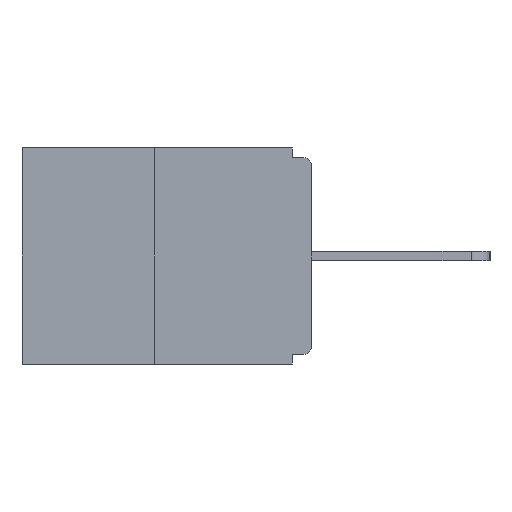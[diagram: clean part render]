
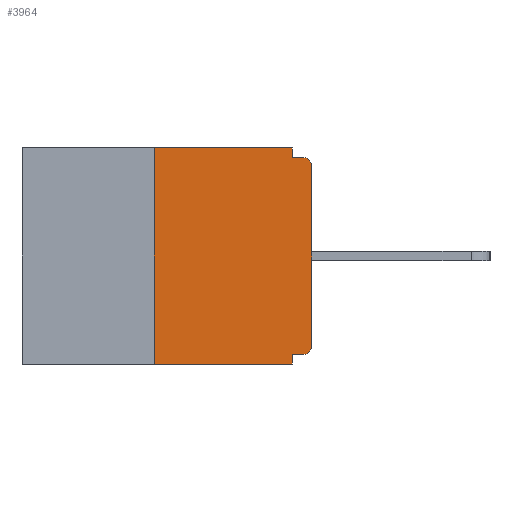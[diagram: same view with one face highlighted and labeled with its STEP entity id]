
A CAD part, left-side view. The second image highlights one B-rep face of the part: STEP entity #3964.
In plain terms, the highlighted planar face has unit normal (-1, 0, 0).
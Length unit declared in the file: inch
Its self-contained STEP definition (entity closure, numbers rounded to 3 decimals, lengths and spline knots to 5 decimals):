
#217 = ORIENTED_EDGE ( 'NONE', *, *, #3717, .T. ) ;
#448 = DIRECTION ( 'NONE',  ( 0., 0., 1. ) ) ;
#612 = VERTEX_POINT ( 'NONE', #13465 ) ;
#772 = LINE ( 'NONE', #8104, #11012 ) ;
#862 = CIRCLE ( 'NONE', #11757, 0.015 ) ;
#958 = CARTESIAN_POINT ( 'NONE',  ( 0., 0., -0.015 ) ) ;
#1286 = VERTEX_POINT ( 'NONE', #6840 ) ;
#1301 = DIRECTION ( 'NONE',  ( 0., -1., 0. ) ) ;
#1333 = CARTESIAN_POINT ( 'NONE',  ( 0., 0.46, 0. ) ) ;
#1517 = ORIENTED_EDGE ( 'NONE', *, *, #14746, .T. ) ;
#1579 = EDGE_CURVE ( 'NONE', #1286, #2035, #12419, .T. ) ;
#2035 = VERTEX_POINT ( 'NONE', #4166 ) ;
#2094 = VECTOR ( 'NONE', #10091, 39.37008 ) ;
#2253 = VERTEX_POINT ( 'NONE', #12683 ) ;
#2357 = LINE ( 'NONE', #7444, #13769 ) ;
#2391 = LINE ( 'NONE', #958, #8960 ) ;
#2914 = ORIENTED_EDGE ( 'NONE', *, *, #11881, .T. ) ;
#3104 = CIRCLE ( 'NONE', #14000, 0.015 ) ;
#3200 = CARTESIAN_POINT ( 'NONE',  ( 0., 0.031, -0.343 ) ) ;
#3345 = DIRECTION ( 'NONE',  ( 0., 0., -1. ) ) ;
#3346 = ORIENTED_EDGE ( 'NONE', *, *, #9229, .F. ) ;
#3465 = DIRECTION ( 'NONE',  ( 0., 0., -1. ) ) ;
#3518 = DIRECTION ( 'NONE',  ( 0., 1., 0. ) ) ;
#3717 = EDGE_CURVE ( 'NONE', #7398, #5540, #3104, .T. ) ;
#3964 = ADVANCED_FACE ( 'NONE', ( #6450 ), #9838, .F. ) ;
#3977 = DIRECTION ( 'NONE',  ( 1., 0., 0. ) ) ;
#4166 = CARTESIAN_POINT ( 'NONE',  ( 0., 0.25, 0. ) ) ;
#4636 = EDGE_CURVE ( 'NONE', #5840, #9240, #13040, .T. ) ;
#4698 = DIRECTION ( 'NONE',  ( -1., 0., 0. ) ) ;
#4813 = CARTESIAN_POINT ( 'NONE',  ( 0., 0., -0.313 ) ) ;
#5268 = CARTESIAN_POINT ( 'NONE',  ( 0., 0., 0. ) ) ;
#5517 = AXIS2_PLACEMENT_3D ( 'NONE', #1333, #3977, #7473 ) ;
#5540 = VERTEX_POINT ( 'NONE', #6209 ) ;
#5823 = EDGE_CURVE ( 'NONE', #2035, #612, #2357, .T. ) ;
#5828 = DIRECTION ( 'NONE',  ( 0., 0., -1. ) ) ;
#5840 = VERTEX_POINT ( 'NONE', #7360 ) ;
#6087 = ORIENTED_EDGE ( 'NONE', *, *, #4636, .F. ) ;
#6209 = CARTESIAN_POINT ( 'NONE',  ( 0., 0.015, -0.015 ) ) ;
#6450 = FACE_OUTER_BOUND ( 'NONE', #9430, .T. ) ;
#6600 = EDGE_CURVE ( 'NONE', #9240, #2253, #9225, .T. ) ;
#6840 = CARTESIAN_POINT ( 'NONE',  ( 0., 0.25, -0.343 ) ) ;
#7049 = DIRECTION ( 'NONE',  ( -1., 0., 0. ) ) ;
#7360 = CARTESIAN_POINT ( 'NONE',  ( 0., 0.015, -0.328 ) ) ;
#7398 = VERTEX_POINT ( 'NONE', #13132 ) ;
#7444 = CARTESIAN_POINT ( 'NONE',  ( 0., 0.46, 0. ) ) ;
#7473 = DIRECTION ( 'NONE',  ( 0., 0., -1. ) ) ;
#8104 = CARTESIAN_POINT ( 'NONE',  ( 0., 0.46, -0.343 ) ) ;
#8343 = CARTESIAN_POINT ( 'NONE',  ( 0., 0.031, -0.015 ) ) ;
#8660 = EDGE_CURVE ( 'NONE', #1286, #2253, #772, .T. ) ;
#8960 = VECTOR ( 'NONE', #10716, 39.37008 ) ;
#9225 = LINE ( 'NONE', #3200, #10509 ) ;
#9229 = EDGE_CURVE ( 'NONE', #612, #12120, #11991, .T. ) ;
#9240 = VERTEX_POINT ( 'NONE', #14378 ) ;
#9430 = EDGE_LOOP ( 'NONE', ( #12361, #12157, #10795, #13089, #6087, #1517, #2914, #217, #12914, #3346 ) ) ;
#9838 = PLANE ( 'NONE',  #5517 ) ;
#10091 = DIRECTION ( 'NONE',  ( 0., 0., 1. ) ) ;
#10509 = VECTOR ( 'NONE', #3345, 39.37008 ) ;
#10691 = VECTOR ( 'NONE', #3518, 39.37008 ) ;
#10716 = DIRECTION ( 'NONE',  ( 0., -1., 0. ) ) ;
#10795 = ORIENTED_EDGE ( 'NONE', *, *, #8660, .T. ) ;
#10970 = LINE ( 'NONE', #5268, #2094 ) ;
#11012 = VECTOR ( 'NONE', #15140, 39.37008 ) ;
#11322 = CARTESIAN_POINT ( 'NONE',  ( 0., 0.25, 0. ) ) ;
#11757 = AXIS2_PLACEMENT_3D ( 'NONE', #13210, #7049, #3465 ) ;
#11881 = EDGE_CURVE ( 'NONE', #13106, #7398, #10970, .T. ) ;
#11991 = LINE ( 'NONE', #14145, #13049 ) ;
#12047 = EDGE_CURVE ( 'NONE', #12120, #5540, #2391, .T. ) ;
#12120 = VERTEX_POINT ( 'NONE', #8343 ) ;
#12157 = ORIENTED_EDGE ( 'NONE', *, *, #1579, .F. ) ;
#12361 = ORIENTED_EDGE ( 'NONE', *, *, #5823, .F. ) ;
#12419 = LINE ( 'NONE', #11322, #13646 ) ;
#12683 = CARTESIAN_POINT ( 'NONE',  ( 0., 0.031, -0.343 ) ) ;
#12704 = CARTESIAN_POINT ( 'NONE',  ( 0., 0.015, -0.03 ) ) ;
#12914 = ORIENTED_EDGE ( 'NONE', *, *, #12047, .F. ) ;
#13040 = LINE ( 'NONE', #15474, #10691 ) ;
#13049 = VECTOR ( 'NONE', #5828, 39.37008 ) ;
#13089 = ORIENTED_EDGE ( 'NONE', *, *, #6600, .F. ) ;
#13106 = VERTEX_POINT ( 'NONE', #4813 ) ;
#13132 = CARTESIAN_POINT ( 'NONE',  ( 0., 0., -0.03 ) ) ;
#13210 = CARTESIAN_POINT ( 'NONE',  ( 0., 0.015, -0.313 ) ) ;
#13465 = CARTESIAN_POINT ( 'NONE',  ( 0., 0.031, 0. ) ) ;
#13646 = VECTOR ( 'NONE', #448, 39.37008 ) ;
#13769 = VECTOR ( 'NONE', #1301, 39.37008 ) ;
#14000 = AXIS2_PLACEMENT_3D ( 'NONE', #12704, #4698, #14136 ) ;
#14136 = DIRECTION ( 'NONE',  ( 0., 0., -1. ) ) ;
#14145 = CARTESIAN_POINT ( 'NONE',  ( 0., 0.031, 0. ) ) ;
#14378 = CARTESIAN_POINT ( 'NONE',  ( 0., 0.031, -0.328 ) ) ;
#14746 = EDGE_CURVE ( 'NONE', #5840, #13106, #862, .T. ) ;
#15140 = DIRECTION ( 'NONE',  ( 0., -1., 0. ) ) ;
#15474 = CARTESIAN_POINT ( 'NONE',  ( 0., 0., -0.328 ) ) ;
